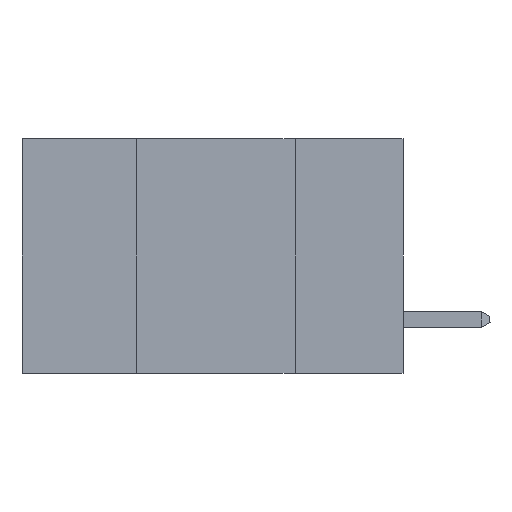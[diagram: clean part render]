
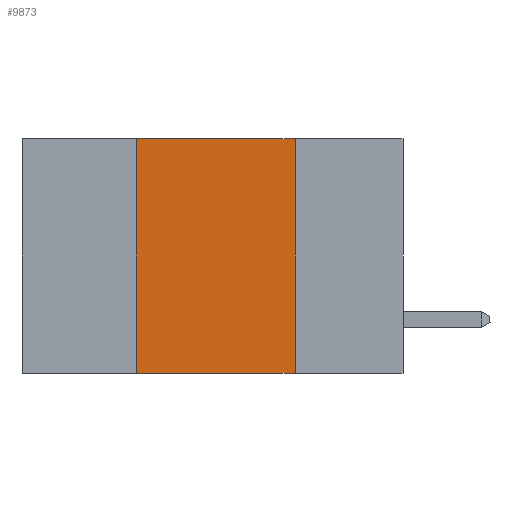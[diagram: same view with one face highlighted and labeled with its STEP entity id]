
A CAD part, left-side view. The second image highlights one B-rep face of the part: STEP entity #9873.
In plain terms, the highlighted planar face has unit normal (-1, 0, 0).
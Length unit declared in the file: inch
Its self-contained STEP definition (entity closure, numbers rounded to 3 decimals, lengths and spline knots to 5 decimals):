
#23 = LINE ( 'NONE', #12050, #11370 ) ;
#1999 = LINE ( 'NONE', #8321, #9172 ) ;
#2327 = EDGE_CURVE ( 'NONE', #7155, #14238, #23, .T. ) ;
#2768 = ORIENTED_EDGE ( 'NONE', *, *, #5155, .T. ) ;
#3121 = AXIS2_PLACEMENT_3D ( 'NONE', #12627, #12854, #15265 ) ;
#3150 = DIRECTION ( 'NONE',  ( 0., -1., 0. ) ) ;
#3726 = LINE ( 'NONE', #9067, #4489 ) ;
#4219 = PLANE ( 'NONE',  #3121 ) ;
#4489 = VECTOR ( 'NONE', #3150, 39.37008 ) ;
#4673 = CARTESIAN_POINT ( 'NONE',  ( 0., 0.42, -0.37 ) ) ;
#4972 = VERTEX_POINT ( 'NONE', #13115 ) ;
#5155 = EDGE_CURVE ( 'NONE', #7155, #6132, #1999, .T. ) ;
#5605 = DIRECTION ( 'NONE',  ( 0., 0., -1. ) ) ;
#5730 = LINE ( 'NONE', #10339, #11598 ) ;
#6041 = FACE_OUTER_BOUND ( 'NONE', #13195, .T. ) ;
#6132 = VERTEX_POINT ( 'NONE', #7359 ) ;
#7155 = VERTEX_POINT ( 'NONE', #4673 ) ;
#7359 = CARTESIAN_POINT ( 'NONE',  ( 0., 0.17, -0.37 ) ) ;
#8321 = CARTESIAN_POINT ( 'NONE',  ( 0., 0.6, -0.37 ) ) ;
#9067 = CARTESIAN_POINT ( 'NONE',  ( 0., 0.6, 0. ) ) ;
#9172 = VECTOR ( 'NONE', #9525, 39.37008 ) ;
#9390 = ORIENTED_EDGE ( 'NONE', *, *, #11177, .F. ) ;
#9525 = DIRECTION ( 'NONE',  ( 0., -1., 0. ) ) ;
#9712 = ORIENTED_EDGE ( 'NONE', *, *, #2327, .F. ) ;
#9873 = ADVANCED_FACE ( 'NONE', ( #6041 ), #4219, .F. ) ;
#10154 = CARTESIAN_POINT ( 'NONE',  ( 0., 0.42, 0. ) ) ;
#10259 = DIRECTION ( 'NONE',  ( 0., 0., 1. ) ) ;
#10339 = CARTESIAN_POINT ( 'NONE',  ( 0., 0.17, 0. ) ) ;
#10532 = ORIENTED_EDGE ( 'NONE', *, *, #14693, .F. ) ;
#11177 = EDGE_CURVE ( 'NONE', #14238, #4972, #3726, .T. ) ;
#11370 = VECTOR ( 'NONE', #10259, 39.37008 ) ;
#11598 = VECTOR ( 'NONE', #5605, 39.37008 ) ;
#12050 = CARTESIAN_POINT ( 'NONE',  ( 0., 0.42, 0. ) ) ;
#12627 = CARTESIAN_POINT ( 'NONE',  ( 0., 0.6, 0. ) ) ;
#12854 = DIRECTION ( 'NONE',  ( 1., 0., 0. ) ) ;
#13115 = CARTESIAN_POINT ( 'NONE',  ( 0., 0.17, 0. ) ) ;
#13195 = EDGE_LOOP ( 'NONE', ( #10532, #9390, #9712, #2768 ) ) ;
#14238 = VERTEX_POINT ( 'NONE', #10154 ) ;
#14693 = EDGE_CURVE ( 'NONE', #4972, #6132, #5730, .T. ) ;
#15265 = DIRECTION ( 'NONE',  ( 0., 0., -1. ) ) ;
